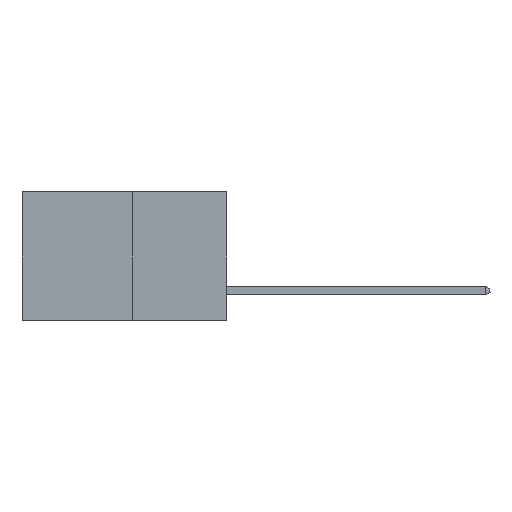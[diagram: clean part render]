
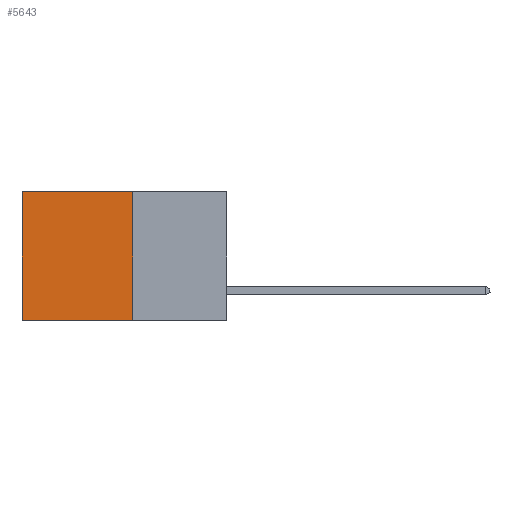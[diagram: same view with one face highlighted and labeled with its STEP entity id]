
A CAD part, left-side view. The second image highlights one B-rep face of the part: STEP entity #5643.
In plain terms, the highlighted planar face has unit normal (-1, 0, 0).
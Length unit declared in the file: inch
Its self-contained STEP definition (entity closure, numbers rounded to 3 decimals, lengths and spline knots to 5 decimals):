
#421 = DIRECTION ( 'NONE',  ( 0., 0., -1. ) ) ;
#1632 = VERTEX_POINT ( 'NONE', #10365 ) ;
#1974 = ORIENTED_EDGE ( 'NONE', *, *, #6100, .F. ) ;
#2250 = EDGE_CURVE ( 'NONE', #4955, #8063, #13351, .T. ) ;
#3384 = CARTESIAN_POINT ( 'NONE',  ( 0.277, 0.27, 0. ) ) ;
#4309 = FACE_OUTER_BOUND ( 'NONE', #12907, .T. ) ;
#4649 = CARTESIAN_POINT ( 'NONE',  ( 0.277, 0.59, -0.37 ) ) ;
#4866 = EDGE_CURVE ( 'NONE', #8942, #4955, #12882, .T. ) ;
#4955 = VERTEX_POINT ( 'NONE', #10468 ) ;
#5439 = DIRECTION ( 'NONE',  ( 0., 0., -1. ) ) ;
#5643 = ADVANCED_FACE ( 'NONE', ( #4309 ), #9471, .F. ) ;
#6089 = VECTOR ( 'NONE', #12666, 39.37008 ) ;
#6100 = EDGE_CURVE ( 'NONE', #1632, #8063, #13490, .T. ) ;
#6312 = CARTESIAN_POINT ( 'NONE',  ( 0.277, 0.59, -0.37 ) ) ;
#7306 = DIRECTION ( 'NONE',  ( 1., 0., 0. ) ) ;
#8063 = VERTEX_POINT ( 'NONE', #4649 ) ;
#8366 = CARTESIAN_POINT ( 'NONE',  ( 0.277, 0.27, -0.37 ) ) ;
#8727 = ORIENTED_EDGE ( 'NONE', *, *, #14258, .F. ) ;
#8942 = VERTEX_POINT ( 'NONE', #3384 ) ;
#9016 = LINE ( 'NONE', #8366, #6089 ) ;
#9471 = PLANE ( 'NONE',  #13759 ) ;
#10089 = VECTOR ( 'NONE', #14103, 39.37008 ) ;
#10365 = CARTESIAN_POINT ( 'NONE',  ( 0.277, 0.27, -0.37 ) ) ;
#10468 = CARTESIAN_POINT ( 'NONE',  ( 0.277, 0.59, 0. ) ) ;
#11726 = VECTOR ( 'NONE', #12303, 39.37008 ) ;
#11932 = ORIENTED_EDGE ( 'NONE', *, *, #4866, .T. ) ;
#12152 = CARTESIAN_POINT ( 'NONE',  ( 0.277, 0.27, -0.37 ) ) ;
#12303 = DIRECTION ( 'NONE',  ( 0., 1., 0. ) ) ;
#12666 = DIRECTION ( 'NONE',  ( 0., 0., -1. ) ) ;
#12882 = LINE ( 'NONE', #14285, #10089 ) ;
#12907 = EDGE_LOOP ( 'NONE', ( #13060, #1974, #8727, #11932 ) ) ;
#13060 = ORIENTED_EDGE ( 'NONE', *, *, #2250, .T. ) ;
#13351 = LINE ( 'NONE', #6312, #13664 ) ;
#13490 = LINE ( 'NONE', #12152, #11726 ) ;
#13664 = VECTOR ( 'NONE', #5439, 39.37008 ) ;
#13708 = CARTESIAN_POINT ( 'NONE',  ( 0.277, 0.27, -0.37 ) ) ;
#13759 = AXIS2_PLACEMENT_3D ( 'NONE', #13708, #7306, #421 ) ;
#14103 = DIRECTION ( 'NONE',  ( 0., 1., 0. ) ) ;
#14258 = EDGE_CURVE ( 'NONE', #8942, #1632, #9016, .T. ) ;
#14285 = CARTESIAN_POINT ( 'NONE',  ( 0.277, 0.27, 0. ) ) ;
